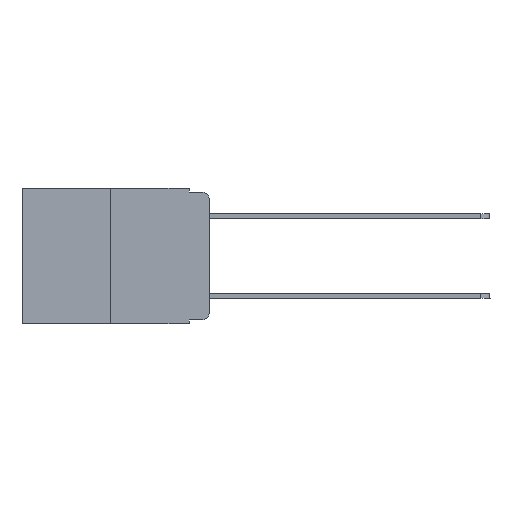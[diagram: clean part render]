
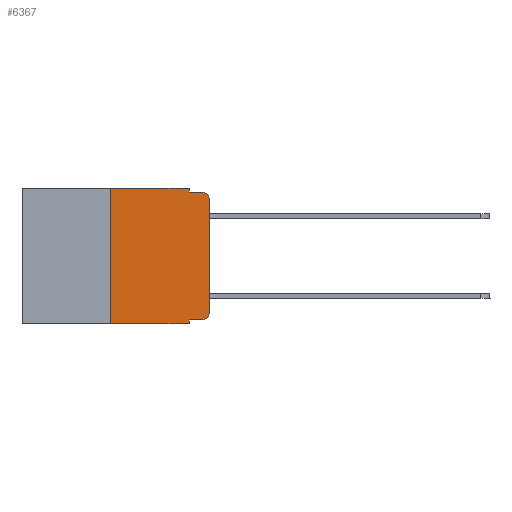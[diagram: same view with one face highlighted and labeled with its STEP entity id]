
A CAD part, left-side view. The second image highlights one B-rep face of the part: STEP entity #6367.
In plain terms, the highlighted planar face has unit normal (-1, 0, 0).
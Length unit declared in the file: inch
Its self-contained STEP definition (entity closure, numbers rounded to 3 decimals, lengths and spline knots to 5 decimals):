
#19 = EDGE_CURVE ( 'NONE', #18687, #19504, #1638, .T. ) ;
#177 = CARTESIAN_POINT ( 'NONE',  ( 0., 0.051, -0.01 ) ) ;
#412 = VECTOR ( 'NONE', #10426, 39.37008 ) ;
#880 = CARTESIAN_POINT ( 'NONE',  ( 0., 0.051, -0.343 ) ) ;
#982 = CARTESIAN_POINT ( 'NONE',  ( 0., 0.25, -0.343 ) ) ;
#1213 = ORIENTED_EDGE ( 'NONE', *, *, #12628, .T. ) ;
#1571 = DIRECTION ( 'NONE',  ( 0., 0., -1. ) ) ;
#1580 = DIRECTION ( 'NONE',  ( 0., 0., 1. ) ) ;
#1638 = LINE ( 'NONE', #17828, #5708 ) ;
#1942 = CIRCLE ( 'NONE', #6664, 0.02 ) ;
#2211 = LINE ( 'NONE', #2311, #6492 ) ;
#2311 = CARTESIAN_POINT ( 'NONE',  ( 0., 0.473, -0.343 ) ) ;
#2405 = VERTEX_POINT ( 'NONE', #9522 ) ;
#2515 = AXIS2_PLACEMENT_3D ( 'NONE', #11292, #5150, #1571 ) ;
#2595 = DIRECTION ( 'NONE',  ( -1., 0., 0. ) ) ;
#2903 = CARTESIAN_POINT ( 'NONE',  ( 0., 0.25, 0. ) ) ;
#3098 = CARTESIAN_POINT ( 'NONE',  ( 0., 0.051, -0.01 ) ) ;
#3133 = VERTEX_POINT ( 'NONE', #15259 ) ;
#3454 = ORIENTED_EDGE ( 'NONE', *, *, #16850, .T. ) ;
#3495 = CARTESIAN_POINT ( 'NONE',  ( 0., 0.051, 0. ) ) ;
#3695 = LINE ( 'NONE', #6564, #5492 ) ;
#3905 = ORIENTED_EDGE ( 'NONE', *, *, #11591, .F. ) ;
#3931 = VERTEX_POINT ( 'NONE', #13842 ) ;
#3936 = VECTOR ( 'NONE', #9243, 39.37008 ) ;
#3971 = LINE ( 'NONE', #5874, #412 ) ;
#4137 = ORIENTED_EDGE ( 'NONE', *, *, #19, .F. ) ;
#4155 = VECTOR ( 'NONE', #1580, 39.37008 ) ;
#4471 = CARTESIAN_POINT ( 'NONE',  ( 0., 0.051, -0.333 ) ) ;
#4475 = CARTESIAN_POINT ( 'NONE',  ( 0., 0.25, 0. ) ) ;
#4556 = ORIENTED_EDGE ( 'NONE', *, *, #6538, .T. ) ;
#5106 = EDGE_CURVE ( 'NONE', #18687, #7739, #3695, .T. ) ;
#5150 = DIRECTION ( 'NONE',  ( -1., 0., 0. ) ) ;
#5385 = EDGE_CURVE ( 'NONE', #3931, #2405, #16071, .T. ) ;
#5492 = VECTOR ( 'NONE', #13012, 39.37008 ) ;
#5508 = EDGE_CURVE ( 'NONE', #13218, #3133, #6845, .T. ) ;
#5708 = VECTOR ( 'NONE', #8080, 39.37008 ) ;
#5874 = CARTESIAN_POINT ( 'NONE',  ( 0., 0.051, 0. ) ) ;
#6367 = ADVANCED_FACE ( 'NONE', ( #13130 ), #19585, .F. ) ;
#6492 = VECTOR ( 'NONE', #8751, 39.37008 ) ;
#6517 = ORIENTED_EDGE ( 'NONE', *, *, #5508, .F. ) ;
#6538 = EDGE_CURVE ( 'NONE', #7739, #3931, #8918, .T. ) ;
#6564 = CARTESIAN_POINT ( 'NONE',  ( 0., 0.051, -0.333 ) ) ;
#6664 = AXIS2_PLACEMENT_3D ( 'NONE', #17406, #2595, #13801 ) ;
#6845 = LINE ( 'NONE', #177, #19389 ) ;
#7739 = VERTEX_POINT ( 'NONE', #18393 ) ;
#7862 = ORIENTED_EDGE ( 'NONE', *, *, #11271, .F. ) ;
#7889 = EDGE_LOOP ( 'NONE', ( #14984, #3454, #6517, #7862, #3905, #10797, #1213, #4137, #19115, #4556 ) ) ;
#8080 = DIRECTION ( 'NONE',  ( 0., 0., -1. ) ) ;
#8281 = LINE ( 'NONE', #11663, #9951 ) ;
#8751 = DIRECTION ( 'NONE',  ( 0., -1., 0. ) ) ;
#8790 = EDGE_CURVE ( 'NONE', #15949, #20685, #9023, .T. ) ;
#8918 = CIRCLE ( 'NONE', #2515, 0.02 ) ;
#9023 = LINE ( 'NONE', #2903, #3936 ) ;
#9243 = DIRECTION ( 'NONE',  ( 0., 0., 1. ) ) ;
#9306 = VERTEX_POINT ( 'NONE', #3495 ) ;
#9399 = DIRECTION ( 'NONE',  ( 0., 0., -1. ) ) ;
#9522 = CARTESIAN_POINT ( 'NONE',  ( 0., 0., -0.03 ) ) ;
#9951 = VECTOR ( 'NONE', #13250, 39.37008 ) ;
#10124 = DIRECTION ( 'NONE',  ( 0., -1., 0. ) ) ;
#10426 = DIRECTION ( 'NONE',  ( 0., 0., -1. ) ) ;
#10797 = ORIENTED_EDGE ( 'NONE', *, *, #8790, .F. ) ;
#11271 = EDGE_CURVE ( 'NONE', #9306, #13218, #3971, .T. ) ;
#11292 = CARTESIAN_POINT ( 'NONE',  ( 0., 0.02, -0.313 ) ) ;
#11591 = EDGE_CURVE ( 'NONE', #20685, #9306, #8281, .T. ) ;
#11663 = CARTESIAN_POINT ( 'NONE',  ( 0., 0.473, 0. ) ) ;
#12628 = EDGE_CURVE ( 'NONE', #15949, #19504, #2211, .T. ) ;
#13012 = DIRECTION ( 'NONE',  ( 0., -1., 0. ) ) ;
#13130 = FACE_OUTER_BOUND ( 'NONE', #7889, .T. ) ;
#13218 = VERTEX_POINT ( 'NONE', #3098 ) ;
#13250 = DIRECTION ( 'NONE',  ( 0., -1., 0. ) ) ;
#13801 = DIRECTION ( 'NONE',  ( 0., 0., -1. ) ) ;
#13842 = CARTESIAN_POINT ( 'NONE',  ( 0., 0., -0.313 ) ) ;
#14041 = CARTESIAN_POINT ( 'NONE',  ( 0., 0.473, 0. ) ) ;
#14984 = ORIENTED_EDGE ( 'NONE', *, *, #5385, .T. ) ;
#15259 = CARTESIAN_POINT ( 'NONE',  ( 0., 0.02, -0.01 ) ) ;
#15949 = VERTEX_POINT ( 'NONE', #982 ) ;
#16071 = LINE ( 'NONE', #17345, #4155 ) ;
#16850 = EDGE_CURVE ( 'NONE', #2405, #3133, #1942, .T. ) ;
#17345 = CARTESIAN_POINT ( 'NONE',  ( 0., 0., 0. ) ) ;
#17406 = CARTESIAN_POINT ( 'NONE',  ( 0., 0.02, -0.03 ) ) ;
#17550 = DIRECTION ( 'NONE',  ( 1., 0., 0. ) ) ;
#17828 = CARTESIAN_POINT ( 'NONE',  ( 0., 0.051, 0. ) ) ;
#18393 = CARTESIAN_POINT ( 'NONE',  ( 0., 0.02, -0.333 ) ) ;
#18687 = VERTEX_POINT ( 'NONE', #4471 ) ;
#18728 = AXIS2_PLACEMENT_3D ( 'NONE', #14041, #17550, #9399 ) ;
#19115 = ORIENTED_EDGE ( 'NONE', *, *, #5106, .T. ) ;
#19389 = VECTOR ( 'NONE', #10124, 39.37008 ) ;
#19504 = VERTEX_POINT ( 'NONE', #880 ) ;
#19585 = PLANE ( 'NONE',  #18728 ) ;
#20685 = VERTEX_POINT ( 'NONE', #4475 ) ;
